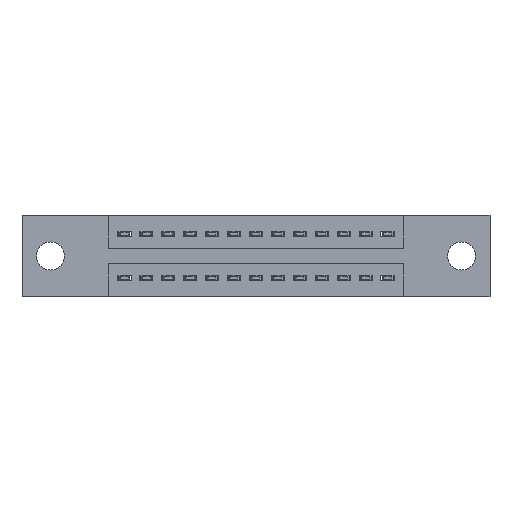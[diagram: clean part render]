
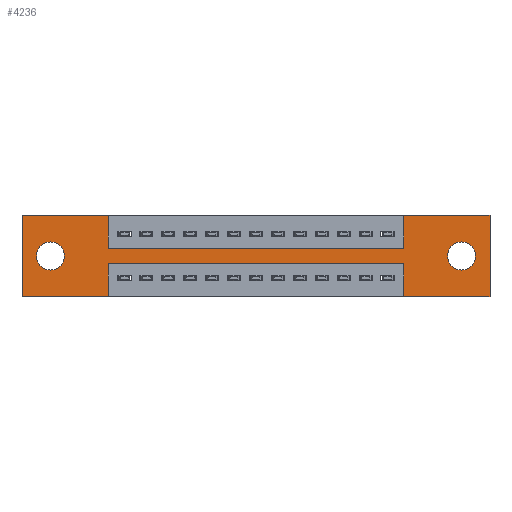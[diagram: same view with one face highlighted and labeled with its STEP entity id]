
A CAD part, front view. The second image highlights one B-rep face of the part: STEP entity #4236.
In plain terms, the highlighted planar face has unit normal (0, -1, 0).
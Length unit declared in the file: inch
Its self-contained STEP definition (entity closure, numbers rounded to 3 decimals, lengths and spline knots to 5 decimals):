
#11 = CARTESIAN_POINT ( 'NONE',  ( 0.3925, 0., -0.22 ) ) ;
#296 = VECTOR ( 'NONE', #3997, 39.37008 ) ;
#338 = VERTEX_POINT ( 'NONE', #3137 ) ;
#358 = DIRECTION ( 'NONE',  ( 0., 0., 1. ) ) ;
#566 = DIRECTION ( 'NONE',  ( -1., 0., 0. ) ) ;
#750 = VERTEX_POINT ( 'NONE', #4935 ) ;
#861 = VERTEX_POINT ( 'NONE', #2637 ) ;
#862 = EDGE_CURVE ( 'NONE', #2712, #13459, #12573, .T. ) ;
#1466 = ORIENTED_EDGE ( 'NONE', *, *, #11232, .T. ) ;
#1478 = ORIENTED_EDGE ( 'NONE', *, *, #2925, .T. ) ;
#1533 = DIRECTION ( 'NONE',  ( 0., 0., 1. ) ) ;
#1554 = EDGE_LOOP ( 'NONE', ( #1614, #1627 ) ) ;
#1614 = ORIENTED_EDGE ( 'NONE', *, *, #12108, .T. ) ;
#1627 = ORIENTED_EDGE ( 'NONE', *, *, #5877, .T. ) ;
#1648 = FACE_BOUND ( 'NONE', #1554, .T. ) ;
#1664 = VERTEX_POINT ( 'NONE', #4372 ) ;
#1700 = ORIENTED_EDGE ( 'NONE', *, *, #8679, .F. ) ;
#1770 = VECTOR ( 'NONE', #3182, 39.37008 ) ;
#1853 = EDGE_CURVE ( 'NONE', #4955, #11299, #5723, .T. ) ;
#1863 = ORIENTED_EDGE ( 'NONE', *, *, #2601, .F. ) ;
#1871 = VECTOR ( 'NONE', #9706, 39.37008 ) ;
#1887 = DIRECTION ( 'NONE',  ( 0., 0., -1. ) ) ;
#1901 = DIRECTION ( 'NONE',  ( 0., -1., 0. ) ) ;
#1953 = CARTESIAN_POINT ( 'NONE',  ( 0., 0., -0.37 ) ) ;
#2009 = ORIENTED_EDGE ( 'NONE', *, *, #5545, .F. ) ;
#2032 = ORIENTED_EDGE ( 'NONE', *, *, #10947, .F. ) ;
#2115 = CIRCLE ( 'NONE', #8278, 0.064 ) ;
#2186 = ORIENTED_EDGE ( 'NONE', *, *, #1853, .F. ) ;
#2196 = ORIENTED_EDGE ( 'NONE', *, *, #10500, .F. ) ;
#2241 = ORIENTED_EDGE ( 'NONE', *, *, #8423, .F. ) ;
#2251 = CARTESIAN_POINT ( 'NONE',  ( 2.135, 0., -0.37 ) ) ;
#2336 = ORIENTED_EDGE ( 'NONE', *, *, #3071, .F. ) ;
#2372 = ORIENTED_EDGE ( 'NONE', *, *, #3817, .F. ) ;
#2383 = ORIENTED_EDGE ( 'NONE', *, *, #4086, .F. ) ;
#2395 = ORIENTED_EDGE ( 'NONE', *, *, #862, .F. ) ;
#2488 = VERTEX_POINT ( 'NONE', #3141 ) ;
#2531 = ORIENTED_EDGE ( 'NONE', *, *, #13777, .F. ) ;
#2574 = PLANE ( 'NONE',  #9557 ) ;
#2601 = EDGE_CURVE ( 'NONE', #2488, #6025, #5520, .T. ) ;
#2637 = CARTESIAN_POINT ( 'NONE',  ( 1.7425, 0., -0.15 ) ) ;
#2684 = DIRECTION ( 'NONE',  ( 0., 0., -1. ) ) ;
#2712 = VERTEX_POINT ( 'NONE', #11337 ) ;
#2791 = DIRECTION ( 'NONE',  ( -1., 0., 0. ) ) ;
#2806 = VECTOR ( 'NONE', #6101, 39.37008 ) ;
#2925 = EDGE_CURVE ( 'NONE', #13181, #3943, #9654, .T. ) ;
#2986 = CARTESIAN_POINT ( 'NONE',  ( 0., 0., 0. ) ) ;
#3071 = EDGE_CURVE ( 'NONE', #338, #861, #13142, .T. ) ;
#3137 = CARTESIAN_POINT ( 'NONE',  ( 0.3925, 0., -0.15 ) ) ;
#3141 = CARTESIAN_POINT ( 'NONE',  ( 1.7425, 0., -0.22 ) ) ;
#3182 = DIRECTION ( 'NONE',  ( 1., 0., 0. ) ) ;
#3776 = LINE ( 'NONE', #2986, #296 ) ;
#3779 = VECTOR ( 'NONE', #13848, 39.37008 ) ;
#3797 = VERTEX_POINT ( 'NONE', #5311 ) ;
#3817 = EDGE_CURVE ( 'NONE', #11171, #338, #8996, .T. ) ;
#3943 = VERTEX_POINT ( 'NONE', #7453 ) ;
#3997 = DIRECTION ( 'NONE',  ( 1., 0., 0. ) ) ;
#4086 = EDGE_CURVE ( 'NONE', #13459, #11171, #3776, .T. ) ;
#4236 = ADVANCED_FACE ( 'NONE', ( #9930, #1648, #12955 ), #2574, .T. ) ;
#4372 = CARTESIAN_POINT ( 'NONE',  ( 0.3925, 0., -0.37 ) ) ;
#4607 = VERTEX_POINT ( 'NONE', #7788 ) ;
#4745 = LINE ( 'NONE', #7552, #1770 ) ;
#4847 = VECTOR ( 'NONE', #5102, 39.37008 ) ;
#4935 = CARTESIAN_POINT ( 'NONE',  ( 1.7425, 0., 0. ) ) ;
#4955 = VERTEX_POINT ( 'NONE', #11158 ) ;
#5102 = DIRECTION ( 'NONE',  ( -1., 0., 0. ) ) ;
#5311 = CARTESIAN_POINT ( 'NONE',  ( 0.13, 0., -0.121 ) ) ;
#5381 = CARTESIAN_POINT ( 'NONE',  ( 0., 0., 0. ) ) ;
#5520 = LINE ( 'NONE', #11, #4847 ) ;
#5545 = EDGE_CURVE ( 'NONE', #7905, #2488, #8420, .T. ) ;
#5566 = VECTOR ( 'NONE', #13131, 39.37008 ) ;
#5723 = LINE ( 'NONE', #6146, #2806 ) ;
#5825 = LINE ( 'NONE', #9162, #13431 ) ;
#5877 = EDGE_CURVE ( 'NONE', #4607, #3797, #2115, .T. ) ;
#6025 = VERTEX_POINT ( 'NONE', #9589 ) ;
#6101 = DIRECTION ( 'NONE',  ( 0., 0., -1. ) ) ;
#6146 = CARTESIAN_POINT ( 'NONE',  ( 2.135, 0., 0. ) ) ;
#6234 = LINE ( 'NONE', #12325, #8709 ) ;
#6398 = AXIS2_PLACEMENT_3D ( 'NONE', #11203, #11191, #11177 ) ;
#6592 = DIRECTION ( 'NONE',  ( 0., 1., 0. ) ) ;
#6701 = CARTESIAN_POINT ( 'NONE',  ( 1.7425, 0., 0. ) ) ;
#7151 = VECTOR ( 'NONE', #1533, 39.37008 ) ;
#7155 = DIRECTION ( 'NONE',  ( 0., 1., 0. ) ) ;
#7453 = CARTESIAN_POINT ( 'NONE',  ( 2.005, 0., -0.121 ) ) ;
#7552 = CARTESIAN_POINT ( 'NONE',  ( 0., 0., 0. ) ) ;
#7788 = CARTESIAN_POINT ( 'NONE',  ( 0.13, 0., -0.249 ) ) ;
#7859 = VECTOR ( 'NONE', #566, 39.37008 ) ;
#7905 = VERTEX_POINT ( 'NONE', #9864 ) ;
#7967 = EDGE_LOOP ( 'NONE', ( #1466, #1478 ) ) ;
#8278 = AXIS2_PLACEMENT_3D ( 'NONE', #10747, #10733, #10721 ) ;
#8420 = LINE ( 'NONE', #13299, #5566 ) ;
#8423 = EDGE_CURVE ( 'NONE', #861, #750, #13597, .T. ) ;
#8555 = CARTESIAN_POINT ( 'NONE',  ( 0.3925, 0., 0. ) ) ;
#8646 = DIRECTION ( 'NONE',  ( 0., 0., -1. ) ) ;
#8679 = EDGE_CURVE ( 'NONE', #6025, #1664, #5825, .T. ) ;
#8709 = VECTOR ( 'NONE', #2791, 39.37008 ) ;
#8853 = AXIS2_PLACEMENT_3D ( 'NONE', #13263, #7155, #358 ) ;
#8996 = LINE ( 'NONE', #8555, #9322 ) ;
#9162 = CARTESIAN_POINT ( 'NONE',  ( 0.3925, 0., -0.37 ) ) ;
#9322 = VECTOR ( 'NONE', #8646, 39.37008 ) ;
#9557 = AXIS2_PLACEMENT_3D ( 'NONE', #1953, #1901, #1887 ) ;
#9589 = CARTESIAN_POINT ( 'NONE',  ( 0.3925, 0., -0.22 ) ) ;
#9654 = CIRCLE ( 'NONE', #6398, 0.064 ) ;
#9706 = DIRECTION ( 'NONE',  ( 1., 0., 0. ) ) ;
#9864 = CARTESIAN_POINT ( 'NONE',  ( 1.7425, 0., -0.37 ) ) ;
#9930 = FACE_BOUND ( 'NONE', #7967, .T. ) ;
#10345 = EDGE_LOOP ( 'NONE', ( #1700, #1863, #2009, #2032, #2186, #2196, #2241, #2336, #2372, #2383, #2395, #2531 ) ) ;
#10500 = EDGE_CURVE ( 'NONE', #750, #4955, #4745, .T. ) ;
#10557 = LINE ( 'NONE', #12374, #7859 ) ;
#10721 = DIRECTION ( 'NONE',  ( 0., 0., 1. ) ) ;
#10733 = DIRECTION ( 'NONE',  ( 0., 1., 0. ) ) ;
#10747 = CARTESIAN_POINT ( 'NONE',  ( 0.13, 0., -0.185 ) ) ;
#10928 = CIRCLE ( 'NONE', #10975, 0.064 ) ;
#10947 = EDGE_CURVE ( 'NONE', #11299, #7905, #6234, .T. ) ;
#10975 = AXIS2_PLACEMENT_3D ( 'NONE', #12744, #6592, #13762 ) ;
#11044 = CARTESIAN_POINT ( 'NONE',  ( 0.3925, 0., -0.15 ) ) ;
#11158 = CARTESIAN_POINT ( 'NONE',  ( 2.135, 0., 0. ) ) ;
#11171 = VERTEX_POINT ( 'NONE', #13632 ) ;
#11177 = DIRECTION ( 'NONE',  ( 0., 0., -1. ) ) ;
#11191 = DIRECTION ( 'NONE',  ( 0., 1., 0. ) ) ;
#11203 = CARTESIAN_POINT ( 'NONE',  ( 2.005, 0., -0.185 ) ) ;
#11232 = EDGE_CURVE ( 'NONE', #3943, #13181, #10928, .T. ) ;
#11299 = VERTEX_POINT ( 'NONE', #2251 ) ;
#11337 = CARTESIAN_POINT ( 'NONE',  ( 0., 0., -0.37 ) ) ;
#11406 = CIRCLE ( 'NONE', #8853, 0.064 ) ;
#11824 = CARTESIAN_POINT ( 'NONE',  ( 2.005, 0., -0.249 ) ) ;
#11936 = CARTESIAN_POINT ( 'NONE',  ( 0., 0., 0. ) ) ;
#12108 = EDGE_CURVE ( 'NONE', #3797, #4607, #11406, .T. ) ;
#12325 = CARTESIAN_POINT ( 'NONE',  ( 0., 0., -0.37 ) ) ;
#12374 = CARTESIAN_POINT ( 'NONE',  ( 0., 0., -0.37 ) ) ;
#12573 = LINE ( 'NONE', #5381, #7151 ) ;
#12744 = CARTESIAN_POINT ( 'NONE',  ( 2.005, 0., -0.185 ) ) ;
#12955 = FACE_OUTER_BOUND ( 'NONE', #10345, .T. ) ;
#13131 = DIRECTION ( 'NONE',  ( 0., 0., 1. ) ) ;
#13142 = LINE ( 'NONE', #11044, #1871 ) ;
#13181 = VERTEX_POINT ( 'NONE', #11824 ) ;
#13263 = CARTESIAN_POINT ( 'NONE',  ( 0.13, 0., -0.185 ) ) ;
#13299 = CARTESIAN_POINT ( 'NONE',  ( 1.7425, 0., -0.37 ) ) ;
#13431 = VECTOR ( 'NONE', #2684, 39.37008 ) ;
#13459 = VERTEX_POINT ( 'NONE', #11936 ) ;
#13597 = LINE ( 'NONE', #6701, #3779 ) ;
#13632 = CARTESIAN_POINT ( 'NONE',  ( 0.3925, 0., 0. ) ) ;
#13762 = DIRECTION ( 'NONE',  ( 0., 0., -1. ) ) ;
#13777 = EDGE_CURVE ( 'NONE', #1664, #2712, #10557, .T. ) ;
#13848 = DIRECTION ( 'NONE',  ( 0., 0., 1. ) ) ;
